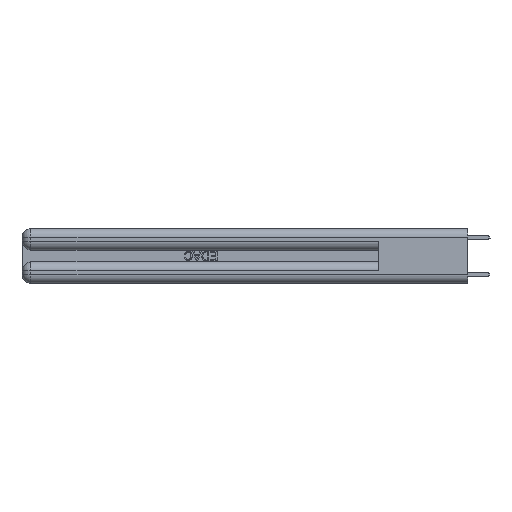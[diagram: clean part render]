
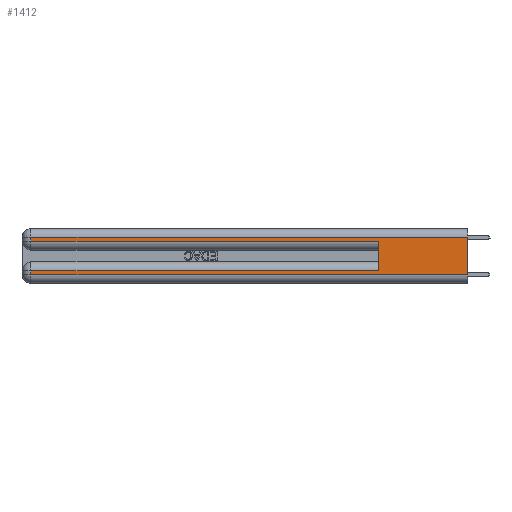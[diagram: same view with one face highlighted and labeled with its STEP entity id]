
A CAD part, left-side view. The second image highlights one B-rep face of the part: STEP entity #1412.
In plain terms, the highlighted planar face has unit normal (-1, 0, 0).
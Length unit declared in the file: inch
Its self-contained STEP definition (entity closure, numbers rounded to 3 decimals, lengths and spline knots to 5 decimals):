
#58 = DIRECTION ( 'NONE',  ( 0., 0., -1. ) ) ;
#910 = VERTEX_POINT ( 'NONE', #2672 ) ;
#1243 = CARTESIAN_POINT ( 'NONE',  ( 0., 0., 0.06 ) ) ;
#1412 = ADVANCED_FACE ( 'NONE', ( #26305 ), #14264, .F. ) ;
#1639 = VECTOR ( 'NONE', #25878, 39.37008 ) ;
#1925 = CARTESIAN_POINT ( 'NONE',  ( 0., 0., 0.06 ) ) ;
#2672 = CARTESIAN_POINT ( 'NONE',  ( 0., 2.94, 0.285 ) ) ;
#2702 = LINE ( 'NONE', #22379, #15145 ) ;
#2775 = VERTEX_POINT ( 'NONE', #6359 ) ;
#2786 = LINE ( 'NONE', #1925, #1639 ) ;
#2861 = DIRECTION ( 'NONE',  ( 0., 0., -1. ) ) ;
#4575 = LINE ( 'NONE', #5246, #16281 ) ;
#4660 = ORIENTED_EDGE ( 'NONE', *, *, #19943, .T. ) ;
#5139 = ORIENTED_EDGE ( 'NONE', *, *, #21105, .T. ) ;
#5246 = CARTESIAN_POINT ( 'NONE',  ( 0., 0., 0.37 ) ) ;
#5869 = CARTESIAN_POINT ( 'NONE',  ( 0., 0.6, 0.085 ) ) ;
#6078 = LINE ( 'NONE', #8322, #9065 ) ;
#6359 = CARTESIAN_POINT ( 'NONE',  ( 0., 0.6, 0.285 ) ) ;
#7304 = VERTEX_POINT ( 'NONE', #15881 ) ;
#7660 = VECTOR ( 'NONE', #2861, 39.37008 ) ;
#8237 = EDGE_CURVE ( 'NONE', #27563, #910, #19881, .T. ) ;
#8322 = CARTESIAN_POINT ( 'NONE',  ( 0., 0.6, 0.145 ) ) ;
#8661 = LINE ( 'NONE', #12571, #10917 ) ;
#9065 = VECTOR ( 'NONE', #22868, 39.37008 ) ;
#9285 = DIRECTION ( 'NONE',  ( 1., 0., 0. ) ) ;
#10140 = CARTESIAN_POINT ( 'NONE',  ( 0., 2.94, 0.31 ) ) ;
#10917 = VECTOR ( 'NONE', #24595, 39.37008 ) ;
#11221 = CARTESIAN_POINT ( 'NONE',  ( 0., 2.94, 0.37 ) ) ;
#11347 = VECTOR ( 'NONE', #28636, 39.37008 ) ;
#12571 = CARTESIAN_POINT ( 'NONE',  ( 0., 0., 0.31 ) ) ;
#13151 = CARTESIAN_POINT ( 'NONE',  ( 0., 2.94, 0.085 ) ) ;
#13386 = VERTEX_POINT ( 'NONE', #15841 ) ;
#14264 = PLANE ( 'NONE',  #30378 ) ;
#15145 = VECTOR ( 'NONE', #27203, 39.37008 ) ;
#15554 = LINE ( 'NONE', #17462, #7660 ) ;
#15841 = CARTESIAN_POINT ( 'NONE',  ( 0., 2.94, 0.06 ) ) ;
#15881 = CARTESIAN_POINT ( 'NONE',  ( 0., 0., 0.31 ) ) ;
#16281 = VECTOR ( 'NONE', #58, 39.37008 ) ;
#16656 = CARTESIAN_POINT ( 'NONE',  ( 0., 0., 0.37 ) ) ;
#17462 = CARTESIAN_POINT ( 'NONE',  ( 0., 2.94, 0.37 ) ) ;
#17539 = EDGE_CURVE ( 'NONE', #7304, #17754, #4575, .T. ) ;
#17754 = VERTEX_POINT ( 'NONE', #1243 ) ;
#17871 = ORIENTED_EDGE ( 'NONE', *, *, #30557, .T. ) ;
#17972 = EDGE_CURVE ( 'NONE', #27069, #2775, #6078, .T. ) ;
#18471 = ORIENTED_EDGE ( 'NONE', *, *, #17539, .F. ) ;
#19264 = EDGE_CURVE ( 'NONE', #29652, #13386, #15554, .T. ) ;
#19881 = LINE ( 'NONE', #11221, #22854 ) ;
#19943 = EDGE_CURVE ( 'NONE', #27069, #29652, #2702, .T. ) ;
#20147 = EDGE_LOOP ( 'NONE', ( #18471, #5139, #27213, #17871, #21847, #4660, #26244, #27699 ) ) ;
#21105 = EDGE_CURVE ( 'NONE', #7304, #27563, #8661, .T. ) ;
#21110 = DIRECTION ( 'NONE',  ( 0., 0., -1. ) ) ;
#21847 = ORIENTED_EDGE ( 'NONE', *, *, #17972, .F. ) ;
#22379 = CARTESIAN_POINT ( 'NONE',  ( 0., 0., 0.085 ) ) ;
#22854 = VECTOR ( 'NONE', #27992, 39.37008 ) ;
#22868 = DIRECTION ( 'NONE',  ( 0., 0., 1. ) ) ;
#24077 = LINE ( 'NONE', #28546, #11347 ) ;
#24595 = DIRECTION ( 'NONE',  ( 0., 1., 0. ) ) ;
#25437 = EDGE_CURVE ( 'NONE', #13386, #17754, #2786, .T. ) ;
#25878 = DIRECTION ( 'NONE',  ( 0., -1., 0. ) ) ;
#26244 = ORIENTED_EDGE ( 'NONE', *, *, #19264, .T. ) ;
#26305 = FACE_OUTER_BOUND ( 'NONE', #20147, .T. ) ;
#27069 = VERTEX_POINT ( 'NONE', #5869 ) ;
#27203 = DIRECTION ( 'NONE',  ( 0., 1., 0. ) ) ;
#27213 = ORIENTED_EDGE ( 'NONE', *, *, #8237, .T. ) ;
#27563 = VERTEX_POINT ( 'NONE', #10140 ) ;
#27699 = ORIENTED_EDGE ( 'NONE', *, *, #25437, .T. ) ;
#27992 = DIRECTION ( 'NONE',  ( 0., 0., -1. ) ) ;
#28546 = CARTESIAN_POINT ( 'NONE',  ( 0., 0., 0.285 ) ) ;
#28636 = DIRECTION ( 'NONE',  ( 0., -1., 0. ) ) ;
#29652 = VERTEX_POINT ( 'NONE', #13151 ) ;
#30378 = AXIS2_PLACEMENT_3D ( 'NONE', #16656, #9285, #21110 ) ;
#30557 = EDGE_CURVE ( 'NONE', #910, #2775, #24077, .T. ) ;
